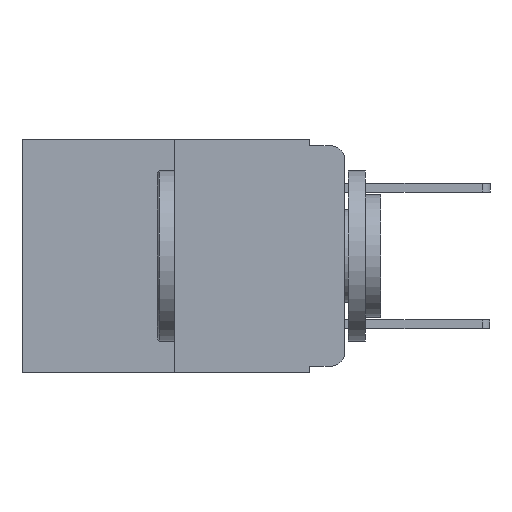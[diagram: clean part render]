
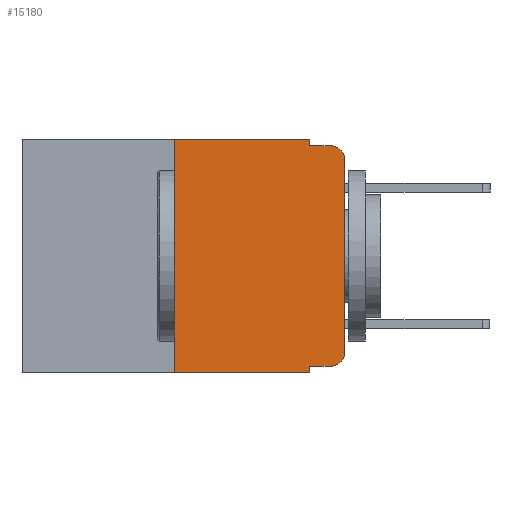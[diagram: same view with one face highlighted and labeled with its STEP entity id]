
A CAD part, left-side view. The second image highlights one B-rep face of the part: STEP entity #15180.
In plain terms, the highlighted planar face has unit normal (-1, 0, 0).
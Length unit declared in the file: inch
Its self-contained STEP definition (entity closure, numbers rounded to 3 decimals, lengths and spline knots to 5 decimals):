
#5 = EDGE_CURVE ( 'NONE', #2694, #6032, #13877, .T. ) ;
#27 = CIRCLE ( 'NONE', #7345, 0.02 ) ;
#428 = EDGE_CURVE ( 'NONE', #2241, #6032, #13857, .T. ) ;
#447 = LINE ( 'NONE', #7799, #15967 ) ;
#486 = CARTESIAN_POINT ( 'NONE',  ( 0., 0., -0.313 ) ) ;
#614 = DIRECTION ( 'NONE',  ( 0., 0., -1. ) ) ;
#686 = EDGE_CURVE ( 'NONE', #8016, #16804, #17874, .T. ) ;
#809 = CARTESIAN_POINT ( 'NONE',  ( 0., 0., 0. ) ) ;
#1047 = EDGE_CURVE ( 'NONE', #1845, #6291, #6812, .T. ) ;
#1744 = CARTESIAN_POINT ( 'NONE',  ( 0., 0.473, -0.343 ) ) ;
#1845 = VERTEX_POINT ( 'NONE', #15890 ) ;
#2241 = VERTEX_POINT ( 'NONE', #12296 ) ;
#2694 = VERTEX_POINT ( 'NONE', #7938 ) ;
#2728 = VECTOR ( 'NONE', #6690, 39.37008 ) ;
#2831 = ORIENTED_EDGE ( 'NONE', *, *, #1047, .F. ) ;
#3347 = VECTOR ( 'NONE', #12468, 39.37008 ) ;
#3470 = DIRECTION ( 'NONE',  ( 0., 0., 1. ) ) ;
#3509 = LINE ( 'NONE', #13651, #14209 ) ;
#3559 = ORIENTED_EDGE ( 'NONE', *, *, #10651, .T. ) ;
#4046 = VERTEX_POINT ( 'NONE', #11163 ) ;
#4508 = CARTESIAN_POINT ( 'NONE',  ( 0., 0., -0.03 ) ) ;
#4583 = DIRECTION ( 'NONE',  ( -1., 0., 0. ) ) ;
#4840 = CARTESIAN_POINT ( 'NONE',  ( 0., 0.02, -0.03 ) ) ;
#4956 = DIRECTION ( 'NONE',  ( 0., -1., 0. ) ) ;
#5222 = CARTESIAN_POINT ( 'NONE',  ( 0., 0.473, 0. ) ) ;
#5419 = AXIS2_PLACEMENT_3D ( 'NONE', #4840, #14975, #6315 ) ;
#5675 = CARTESIAN_POINT ( 'NONE',  ( 0., 0.051, -0.01 ) ) ;
#6032 = VERTEX_POINT ( 'NONE', #10159 ) ;
#6162 = VECTOR ( 'NONE', #614, 39.37008 ) ;
#6200 = LINE ( 'NONE', #5222, #2728 ) ;
#6256 = VERTEX_POINT ( 'NONE', #14932 ) ;
#6291 = VERTEX_POINT ( 'NONE', #17845 ) ;
#6315 = DIRECTION ( 'NONE',  ( 0., 0., -1. ) ) ;
#6555 = ORIENTED_EDGE ( 'NONE', *, *, #11255, .F. ) ;
#6690 = DIRECTION ( 'NONE',  ( 0., -1., 0. ) ) ;
#6812 = LINE ( 'NONE', #5675, #3347 ) ;
#6905 = VECTOR ( 'NONE', #4956, 39.37008 ) ;
#7237 = CARTESIAN_POINT ( 'NONE',  ( 0., 0.473, 0. ) ) ;
#7260 = CARTESIAN_POINT ( 'NONE',  ( 0., 0.25, 0. ) ) ;
#7345 = AXIS2_PLACEMENT_3D ( 'NONE', #13289, #4583, #14738 ) ;
#7490 = ORIENTED_EDGE ( 'NONE', *, *, #686, .T. ) ;
#7799 = CARTESIAN_POINT ( 'NONE',  ( 0., 0.051, 0. ) ) ;
#7938 = CARTESIAN_POINT ( 'NONE',  ( 0., 0.25, -0.343 ) ) ;
#8016 = VERTEX_POINT ( 'NONE', #486 ) ;
#8712 = DIRECTION ( 'NONE',  ( 0., 0., -1. ) ) ;
#9223 = DIRECTION ( 'NONE',  ( 0., 0., -1. ) ) ;
#9321 = EDGE_CURVE ( 'NONE', #2694, #12321, #3509, .T. ) ;
#9322 = DIRECTION ( 'NONE',  ( 0., 0., 1. ) ) ;
#9689 = EDGE_CURVE ( 'NONE', #4046, #8016, #27, .T. ) ;
#10159 = CARTESIAN_POINT ( 'NONE',  ( 0., 0.051, -0.343 ) ) ;
#10651 = EDGE_CURVE ( 'NONE', #2241, #4046, #10788, .T. ) ;
#10757 = ORIENTED_EDGE ( 'NONE', *, *, #428, .F. ) ;
#10788 = LINE ( 'NONE', #17879, #6905 ) ;
#11163 = CARTESIAN_POINT ( 'NONE',  ( 0., 0.02, -0.333 ) ) ;
#11237 = ORIENTED_EDGE ( 'NONE', *, *, #5, .T. ) ;
#11255 = EDGE_CURVE ( 'NONE', #6256, #1845, #447, .T. ) ;
#11873 = EDGE_CURVE ( 'NONE', #16804, #6291, #16588, .T. ) ;
#12018 = ORIENTED_EDGE ( 'NONE', *, *, #11873, .T. ) ;
#12075 = EDGE_CURVE ( 'NONE', #12321, #6256, #6200, .T. ) ;
#12113 = ORIENTED_EDGE ( 'NONE', *, *, #9321, .F. ) ;
#12243 = CARTESIAN_POINT ( 'NONE',  ( 0., 0.051, 0. ) ) ;
#12296 = CARTESIAN_POINT ( 'NONE',  ( 0., 0.051, -0.333 ) ) ;
#12321 = VERTEX_POINT ( 'NONE', #7260 ) ;
#12468 = DIRECTION ( 'NONE',  ( 0., -1., 0. ) ) ;
#13289 = CARTESIAN_POINT ( 'NONE',  ( 0., 0.02, -0.313 ) ) ;
#13344 = FACE_OUTER_BOUND ( 'NONE', #17977, .T. ) ;
#13430 = VECTOR ( 'NONE', #17969, 39.37008 ) ;
#13651 = CARTESIAN_POINT ( 'NONE',  ( 0., 0.25, 0. ) ) ;
#13857 = LINE ( 'NONE', #12243, #6162 ) ;
#13877 = LINE ( 'NONE', #1744, #13430 ) ;
#13918 = ORIENTED_EDGE ( 'NONE', *, *, #12075, .F. ) ;
#14209 = VECTOR ( 'NONE', #3470, 39.37008 ) ;
#14738 = DIRECTION ( 'NONE',  ( 0., 0., -1. ) ) ;
#14932 = CARTESIAN_POINT ( 'NONE',  ( 0., 0.051, 0. ) ) ;
#14975 = DIRECTION ( 'NONE',  ( -1., 0., 0. ) ) ;
#15180 = ADVANCED_FACE ( 'NONE', ( #13344 ), #18699, .F. ) ;
#15890 = CARTESIAN_POINT ( 'NONE',  ( 0., 0.051, -0.01 ) ) ;
#15967 = VECTOR ( 'NONE', #9223, 39.37008 ) ;
#16588 = CIRCLE ( 'NONE', #5419, 0.02 ) ;
#16804 = VERTEX_POINT ( 'NONE', #4508 ) ;
#16972 = VECTOR ( 'NONE', #9322, 39.37008 ) ;
#17020 = ORIENTED_EDGE ( 'NONE', *, *, #9689, .T. ) ;
#17314 = DIRECTION ( 'NONE',  ( 1., 0., 0. ) ) ;
#17420 = AXIS2_PLACEMENT_3D ( 'NONE', #7237, #17314, #8712 ) ;
#17845 = CARTESIAN_POINT ( 'NONE',  ( 0., 0.02, -0.01 ) ) ;
#17874 = LINE ( 'NONE', #809, #16972 ) ;
#17879 = CARTESIAN_POINT ( 'NONE',  ( 0., 0.051, -0.333 ) ) ;
#17969 = DIRECTION ( 'NONE',  ( 0., -1., 0. ) ) ;
#17977 = EDGE_LOOP ( 'NONE', ( #7490, #12018, #2831, #6555, #13918, #12113, #11237, #10757, #3559, #17020 ) ) ;
#18699 = PLANE ( 'NONE',  #17420 ) ;
